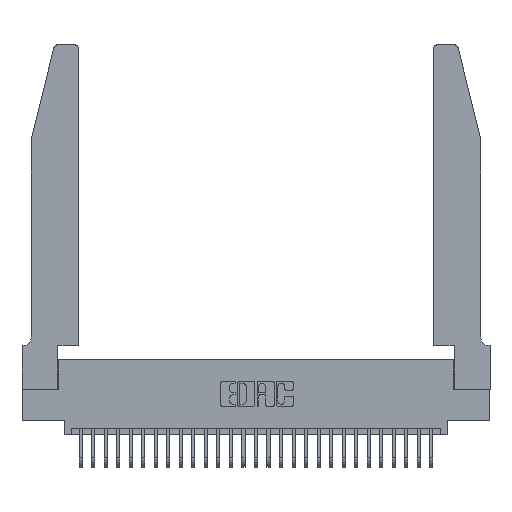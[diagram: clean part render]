
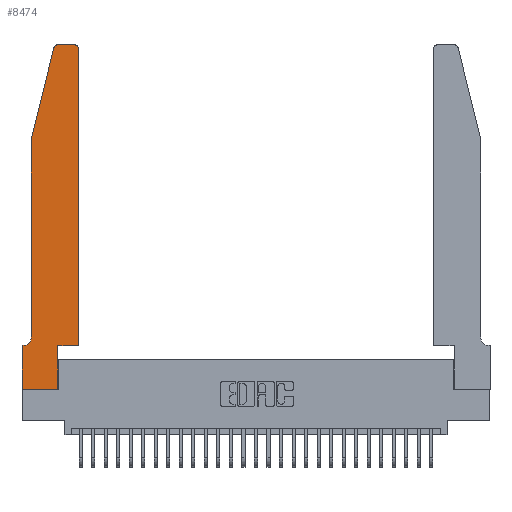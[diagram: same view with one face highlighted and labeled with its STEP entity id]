
A CAD part, top view. The second image highlights one B-rep face of the part: STEP entity #8474.
In plain terms, the highlighted planar face has unit normal (0, 0, 1).
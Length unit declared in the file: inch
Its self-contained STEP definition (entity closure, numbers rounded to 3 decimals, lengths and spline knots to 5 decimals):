
#1087 = CARTESIAN_POINT ( 'NONE',  ( 0.2865, 0.35, 0.37 ) ) ;
#1094 = CARTESIAN_POINT ( 'NONE',  ( 0., 0., 0.37 ) ) ;
#1117 = CARTESIAN_POINT ( 'NONE',  ( 0.4505, 0.35, 0.37 ) ) ;
#1332 = CARTESIAN_POINT ( 'NONE',  ( 0.2865, 0.35, 0.37 ) ) ;
#1589 = LINE ( 'NONE', #1332, #16925 ) ;
#1901 = EDGE_CURVE ( 'NONE', #12498, #8759, #13304, .T. ) ;
#2178 = EDGE_CURVE ( 'NONE', #12248, #17857, #29443, .T. ) ;
#2226 = CARTESIAN_POINT ( 'NONE',  ( 0., 0., 0.37 ) ) ;
#2300 = CARTESIAN_POINT ( 'NONE',  ( 0.2865, 0., 0.37 ) ) ;
#2466 = DIRECTION ( 'NONE',  ( -0.239, -0.971, 0. ) ) ;
#2569 = CARTESIAN_POINT ( 'NONE',  ( 0.0755, 0.35, 0.37 ) ) ;
#3044 = EDGE_LOOP ( 'NONE', ( #30242, #20812, #29028, #13374, #3457, #16577, #30455, #25034, #6593, #20976, #10070, #29268 ) ) ;
#3457 = ORIENTED_EDGE ( 'NONE', *, *, #5086, .T. ) ;
#3901 = EDGE_CURVE ( 'NONE', #8604, #23351, #10198, .T. ) ;
#4429 = EDGE_CURVE ( 'NONE', #9676, #22822, #10907, .T. ) ;
#4730 = DIRECTION ( 'NONE',  ( 1., 0., 0. ) ) ;
#5061 = VECTOR ( 'NONE', #7456, 39.37008 ) ;
#5086 = EDGE_CURVE ( 'NONE', #12661, #24121, #25880, .T. ) ;
#5408 = CARTESIAN_POINT ( 'NONE',  ( 0., 0., 0.37 ) ) ;
#5431 = LINE ( 'NONE', #8729, #23832 ) ;
#6015 = DIRECTION ( 'NONE',  ( 0., 1., 0. ) ) ;
#6102 = VECTOR ( 'NONE', #2466, 39.37008 ) ;
#6250 = AXIS2_PLACEMENT_3D ( 'NONE', #24691, #22126, #12320 ) ;
#6253 = DIRECTION ( 'NONE',  ( -1., 0., 0. ) ) ;
#6593 = ORIENTED_EDGE ( 'NONE', *, *, #7205, .T. ) ;
#7205 = EDGE_CURVE ( 'NONE', #11941, #12248, #1589, .T. ) ;
#7242 = EDGE_CURVE ( 'NONE', #22822, #12498, #19183, .T. ) ;
#7456 = DIRECTION ( 'NONE',  ( -1., 0., 0. ) ) ;
#8073 = EDGE_CURVE ( 'NONE', #23351, #11941, #17315, .T. ) ;
#8474 = ADVANCED_FACE ( 'NONE', ( #15028 ), #24369, .T. ) ;
#8604 = VERTEX_POINT ( 'NONE', #11118 ) ;
#8729 = CARTESIAN_POINT ( 'NONE',  ( 0.0755, 2., 0.37 ) ) ;
#8759 = VERTEX_POINT ( 'NONE', #19881 ) ;
#9182 = DIRECTION ( 'NONE',  ( -1., 0., 0. ) ) ;
#9524 = EDGE_CURVE ( 'NONE', #17857, #9676, #17597, .T. ) ;
#9676 = VERTEX_POINT ( 'NONE', #10108 ) ;
#10070 = ORIENTED_EDGE ( 'NONE', *, *, #9524, .T. ) ;
#10108 = CARTESIAN_POINT ( 'NONE',  ( 0.4505, 2.72, 0.37 ) ) ;
#10198 = LINE ( 'NONE', #5408, #21771 ) ;
#10506 = VECTOR ( 'NONE', #6015, 39.37008 ) ;
#10907 = CIRCLE ( 'NONE', #30115, 0.03 ) ;
#10921 = CARTESIAN_POINT ( 'NONE',  ( 0.4205, 2.75, 0.37 ) ) ;
#11118 = CARTESIAN_POINT ( 'NONE',  ( 0., 0.35, 0.37 ) ) ;
#11941 = VERTEX_POINT ( 'NONE', #2300 ) ;
#12048 = DIRECTION ( 'NONE',  ( 1., 0., 0. ) ) ;
#12248 = VERTEX_POINT ( 'NONE', #1087 ) ;
#12320 = DIRECTION ( 'NONE',  ( 1., 0., 0. ) ) ;
#12498 = VERTEX_POINT ( 'NONE', #17031 ) ;
#12655 = EDGE_CURVE ( 'NONE', #24121, #8604, #22285, .T. ) ;
#12661 = VERTEX_POINT ( 'NONE', #19301 ) ;
#12785 = AXIS2_PLACEMENT_3D ( 'NONE', #19562, #25324, #22020 ) ;
#12931 = EDGE_CURVE ( 'NONE', #29104, #12661, #5431, .T. ) ;
#13304 = CIRCLE ( 'NONE', #12785, 0.03 ) ;
#13374 = ORIENTED_EDGE ( 'NONE', *, *, #12931, .T. ) ;
#13395 = CARTESIAN_POINT ( 'NONE',  ( 0.4505, 0.35, 0.37 ) ) ;
#14414 = DIRECTION ( 'NONE',  ( 1., 0., 0. ) ) ;
#15028 = FACE_OUTER_BOUND ( 'NONE', #3044, .T. ) ;
#15153 = DIRECTION ( 'NONE',  ( 0., -1., 0. ) ) ;
#15906 = DIRECTION ( 'NONE',  ( 0., 0., -1. ) ) ;
#16479 = CARTESIAN_POINT ( 'NONE',  ( 0.0755, 2., 0.37 ) ) ;
#16577 = ORIENTED_EDGE ( 'NONE', *, *, #12655, .T. ) ;
#16713 = CARTESIAN_POINT ( 'NONE',  ( 0.4205, 2.72, 0.37 ) ) ;
#16925 = VECTOR ( 'NONE', #23085, 39.37008 ) ;
#17031 = CARTESIAN_POINT ( 'NONE',  ( 0.284, 2.75, 0.37 ) ) ;
#17315 = LINE ( 'NONE', #2226, #27512 ) ;
#17597 = LINE ( 'NONE', #1117, #10506 ) ;
#17857 = VERTEX_POINT ( 'NONE', #13395 ) ;
#18829 = CARTESIAN_POINT ( 'NONE',  ( 0.4505, 0.35, 0.37 ) ) ;
#19183 = LINE ( 'NONE', #23540, #20677 ) ;
#19301 = CARTESIAN_POINT ( 'NONE',  ( 0.0755, 0.42, 0.37 ) ) ;
#19562 = CARTESIAN_POINT ( 'NONE',  ( 0.284, 2.72, 0.37 ) ) ;
#19881 = CARTESIAN_POINT ( 'NONE',  ( 0.25487, 2.72718, 0.37 ) ) ;
#20648 = DIRECTION ( 'NONE',  ( 0., -1., 0. ) ) ;
#20677 = VECTOR ( 'NONE', #9182, 39.37008 ) ;
#20812 = ORIENTED_EDGE ( 'NONE', *, *, #1901, .T. ) ;
#20976 = ORIENTED_EDGE ( 'NONE', *, *, #2178, .T. ) ;
#21217 = CARTESIAN_POINT ( 'NONE',  ( 0.0755, 2., 0.37 ) ) ;
#21468 = LINE ( 'NONE', #21217, #6102 ) ;
#21771 = VECTOR ( 'NONE', #15153, 39.37008 ) ;
#21903 = EDGE_CURVE ( 'NONE', #8759, #29104, #21468, .T. ) ;
#22020 = DIRECTION ( 'NONE',  ( 1., 0., 0. ) ) ;
#22126 = DIRECTION ( 'NONE',  ( 0., 0., 1. ) ) ;
#22285 = LINE ( 'NONE', #2569, #5061 ) ;
#22822 = VERTEX_POINT ( 'NONE', #10921 ) ;
#23085 = DIRECTION ( 'NONE',  ( 0., 1., 0. ) ) ;
#23351 = VERTEX_POINT ( 'NONE', #1094 ) ;
#23540 = CARTESIAN_POINT ( 'NONE',  ( 0.2605, 2.75, 0.37 ) ) ;
#23832 = VECTOR ( 'NONE', #20648, 39.37008 ) ;
#23969 = DIRECTION ( 'NONE',  ( 0., 0., 1. ) ) ;
#24121 = VERTEX_POINT ( 'NONE', #29285 ) ;
#24369 = PLANE ( 'NONE',  #6250 ) ;
#24691 = CARTESIAN_POINT ( 'NONE',  ( 0., 0.35, 0.37 ) ) ;
#25034 = ORIENTED_EDGE ( 'NONE', *, *, #8073, .T. ) ;
#25324 = DIRECTION ( 'NONE',  ( 0., 0., 1. ) ) ;
#25360 = CARTESIAN_POINT ( 'NONE',  ( 0.0055, 0.42, 0.37 ) ) ;
#25880 = CIRCLE ( 'NONE', #29364, 0.07 ) ;
#27512 = VECTOR ( 'NONE', #4730, 39.37008 ) ;
#27944 = VECTOR ( 'NONE', #12048, 39.37008 ) ;
#29028 = ORIENTED_EDGE ( 'NONE', *, *, #21903, .T. ) ;
#29104 = VERTEX_POINT ( 'NONE', #16479 ) ;
#29268 = ORIENTED_EDGE ( 'NONE', *, *, #4429, .T. ) ;
#29285 = CARTESIAN_POINT ( 'NONE',  ( 0.0055, 0.35, 0.37 ) ) ;
#29364 = AXIS2_PLACEMENT_3D ( 'NONE', #25360, #15906, #6253 ) ;
#29443 = LINE ( 'NONE', #18829, #27944 ) ;
#30115 = AXIS2_PLACEMENT_3D ( 'NONE', #16713, #23969, #14414 ) ;
#30242 = ORIENTED_EDGE ( 'NONE', *, *, #7242, .T. ) ;
#30455 = ORIENTED_EDGE ( 'NONE', *, *, #3901, .T. ) ;
